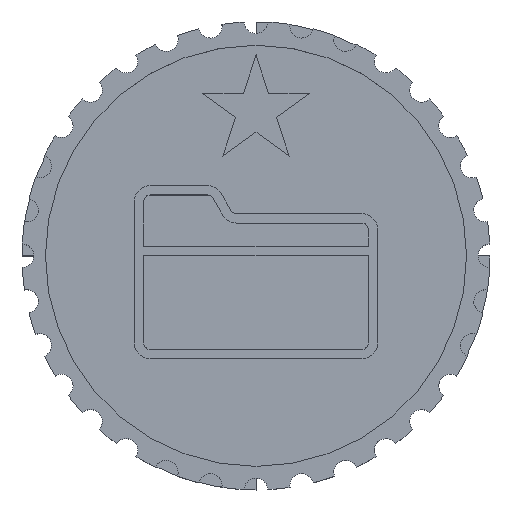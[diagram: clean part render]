
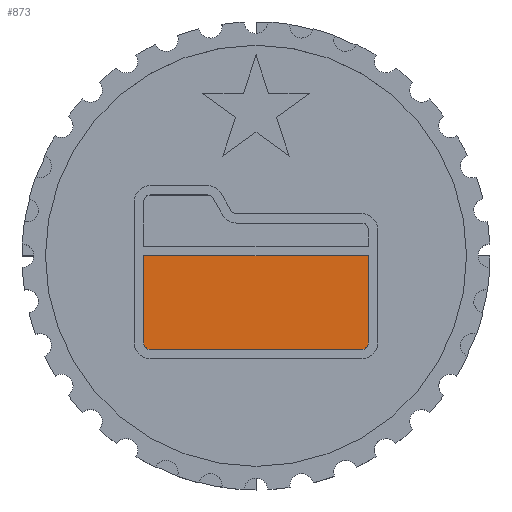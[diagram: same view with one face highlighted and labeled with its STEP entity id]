
A CAD part, top view. The second image highlights one B-rep face of the part: STEP entity #873.
In plain terms, the highlighted planar face has unit normal (0, 0, 1).
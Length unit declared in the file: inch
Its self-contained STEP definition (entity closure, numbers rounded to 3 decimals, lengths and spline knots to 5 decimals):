
#121 = VECTOR ( 'NONE', #4506, 39.37008 ) ;
#285 = ORIENTED_EDGE ( 'NONE', *, *, #5421, .T. ) ;
#513 = AXIS2_PLACEMENT_3D ( 'NONE', #661, #3157, #3616 ) ;
#576 = AXIS2_PLACEMENT_3D ( 'NONE', #5257, #2267, #4354 ) ;
#642 = CARTESIAN_POINT ( 'NONE',  ( -0.3, 0., 0.26063 ) ) ;
#661 = CARTESIAN_POINT ( 'NONE',  ( 0.2825, -0.2325, 0.26063 ) ) ;
#690 = DIRECTION ( 'NONE',  ( 1., 0., 0. ) ) ;
#835 = CARTESIAN_POINT ( 'NONE',  ( 0.2825, -0.25, 0.26063 ) ) ;
#873 = ADVANCED_FACE ( 'NONE', ( #3189 ), #3100, .T. ) ;
#1003 = CARTESIAN_POINT ( 'NONE',  ( 0.3, 0., 0.26063 ) ) ;
#1243 = EDGE_CURVE ( 'NONE', #1270, #2640, #1399, .T. ) ;
#1270 = VERTEX_POINT ( 'NONE', #642 ) ;
#1359 = VECTOR ( 'NONE', #690, 39.37008 ) ;
#1362 = EDGE_CURVE ( 'NONE', #3527, #2640, #5055, .T. ) ;
#1399 = LINE ( 'NONE', #3158, #2728 ) ;
#1429 = ORIENTED_EDGE ( 'NONE', *, *, #4079, .T. ) ;
#1462 = DIRECTION ( 'NONE',  ( 0., 0., 1. ) ) ;
#2267 = DIRECTION ( 'NONE',  ( 0., 0., 1. ) ) ;
#2640 = VERTEX_POINT ( 'NONE', #1003 ) ;
#2701 = DIRECTION ( 'NONE',  ( 1., 0., 0. ) ) ;
#2725 = EDGE_CURVE ( 'NONE', #1270, #3941, #3494, .T. ) ;
#2728 = VECTOR ( 'NONE', #2701, 39.37008 ) ;
#2747 = ORIENTED_EDGE ( 'NONE', *, *, #1243, .F. ) ;
#2771 = VERTEX_POINT ( 'NONE', #3783 ) ;
#2848 = DIRECTION ( 'NONE',  ( 0., 1., 0. ) ) ;
#3100 = PLANE ( 'NONE',  #5503 ) ;
#3131 = DIRECTION ( 'NONE',  ( 1., 0., 0. ) ) ;
#3157 = DIRECTION ( 'NONE',  ( 0., 0., 1. ) ) ;
#3158 = CARTESIAN_POINT ( 'NONE',  ( -0.3, 0., 0.26063 ) ) ;
#3189 = FACE_OUTER_BOUND ( 'NONE', #4879, .T. ) ;
#3281 = LINE ( 'NONE', #4066, #1359 ) ;
#3494 = LINE ( 'NONE', #4088, #121 ) ;
#3527 = VERTEX_POINT ( 'NONE', #4657 ) ;
#3601 = ORIENTED_EDGE ( 'NONE', *, *, #4266, .T. ) ;
#3609 = ORIENTED_EDGE ( 'NONE', *, *, #2725, .T. ) ;
#3616 = DIRECTION ( 'NONE',  ( 1., 0., 0. ) ) ;
#3783 = CARTESIAN_POINT ( 'NONE',  ( -0.2825, -0.25, 0.26063 ) ) ;
#3941 = VERTEX_POINT ( 'NONE', #5104 ) ;
#3988 = CARTESIAN_POINT ( 'NONE',  ( 0., 0., 0.26063 ) ) ;
#4066 = CARTESIAN_POINT ( 'NONE',  ( -0.2825, -0.25, 0.26063 ) ) ;
#4079 = EDGE_CURVE ( 'NONE', #3941, #2771, #4204, .T. ) ;
#4088 = CARTESIAN_POINT ( 'NONE',  ( -0.3, 0.05, 0.26063 ) ) ;
#4089 = ORIENTED_EDGE ( 'NONE', *, *, #1362, .T. ) ;
#4158 = CARTESIAN_POINT ( 'NONE',  ( 0.3, 0.07, 0.26063 ) ) ;
#4204 = CIRCLE ( 'NONE', #576, 0.0175 ) ;
#4266 = EDGE_CURVE ( 'NONE', #2771, #4495, #3281, .T. ) ;
#4354 = DIRECTION ( 'NONE',  ( 1., 0., 0. ) ) ;
#4495 = VERTEX_POINT ( 'NONE', #835 ) ;
#4506 = DIRECTION ( 'NONE',  ( 0., -1., 0. ) ) ;
#4563 = CIRCLE ( 'NONE', #513, 0.0175 ) ;
#4656 = VECTOR ( 'NONE', #2848, 39.37008 ) ;
#4657 = CARTESIAN_POINT ( 'NONE',  ( 0.3, -0.2325, 0.26063 ) ) ;
#4879 = EDGE_LOOP ( 'NONE', ( #4089, #2747, #3609, #1429, #3601, #285 ) ) ;
#5055 = LINE ( 'NONE', #4158, #4656 ) ;
#5104 = CARTESIAN_POINT ( 'NONE',  ( -0.3, -0.2325, 0.26063 ) ) ;
#5257 = CARTESIAN_POINT ( 'NONE',  ( -0.2825, -0.2325, 0.26063 ) ) ;
#5421 = EDGE_CURVE ( 'NONE', #4495, #3527, #4563, .T. ) ;
#5503 = AXIS2_PLACEMENT_3D ( 'NONE', #3988, #1462, #3131 ) ;
